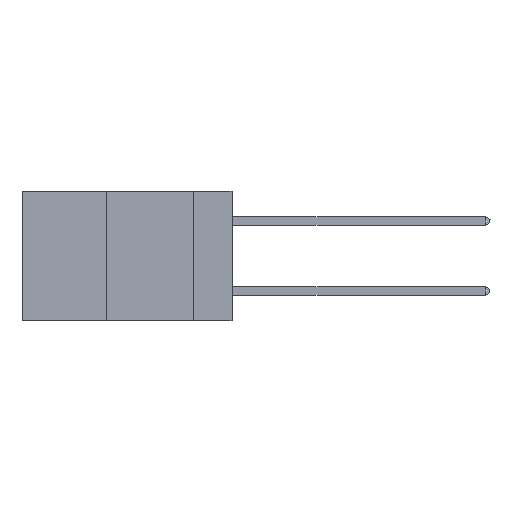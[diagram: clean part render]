
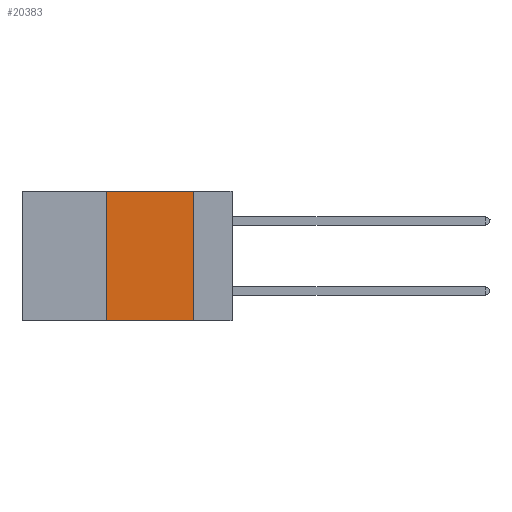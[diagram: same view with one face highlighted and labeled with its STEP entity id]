
A CAD part, left-side view. The second image highlights one B-rep face of the part: STEP entity #20383.
In plain terms, the highlighted planar face has unit normal (-1, 0, 0).
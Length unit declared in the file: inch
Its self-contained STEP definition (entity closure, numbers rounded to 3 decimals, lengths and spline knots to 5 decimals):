
#165 = EDGE_CURVE ( 'NONE', #16418, #5403, #18769, .T. ) ;
#1381 = CARTESIAN_POINT ( 'NONE',  ( 0., 0.6, 0. ) ) ;
#2147 = ORIENTED_EDGE ( 'NONE', *, *, #17951, .F. ) ;
#2774 = CARTESIAN_POINT ( 'NONE',  ( 0., 0.6, -0.37 ) ) ;
#3889 = VECTOR ( 'NONE', #14009, 39.37008 ) ;
#4138 = CARTESIAN_POINT ( 'NONE',  ( 0., 0.11, 0. ) ) ;
#4180 = ORIENTED_EDGE ( 'NONE', *, *, #7829, .F. ) ;
#4671 = VERTEX_POINT ( 'NONE', #11253 ) ;
#5403 = VERTEX_POINT ( 'NONE', #4138 ) ;
#6402 = CARTESIAN_POINT ( 'NONE',  ( 0., 0.11, -0.37 ) ) ;
#6785 = ORIENTED_EDGE ( 'NONE', *, *, #165, .F. ) ;
#6992 = VECTOR ( 'NONE', #8208, 39.37008 ) ;
#7829 = EDGE_CURVE ( 'NONE', #5403, #17338, #13339, .T. ) ;
#8042 = VECTOR ( 'NONE', #8101, 39.37008 ) ;
#8101 = DIRECTION ( 'NONE',  ( 0., 0., 1. ) ) ;
#8208 = DIRECTION ( 'NONE',  ( 0., -1., 0. ) ) ;
#8416 = DIRECTION ( 'NONE',  ( 0., 0., -1. ) ) ;
#8870 = EDGE_CURVE ( 'NONE', #4671, #17338, #15714, .T. ) ;
#9381 = ORIENTED_EDGE ( 'NONE', *, *, #8870, .T. ) ;
#9896 = FACE_OUTER_BOUND ( 'NONE', #21967, .T. ) ;
#10571 = CARTESIAN_POINT ( 'NONE',  ( 0., 0.11, 0. ) ) ;
#11253 = CARTESIAN_POINT ( 'NONE',  ( 0., 0.36, -0.37 ) ) ;
#12671 = CARTESIAN_POINT ( 'NONE',  ( 0., 0.36, 0. ) ) ;
#13225 = LINE ( 'NONE', #16712, #8042 ) ;
#13339 = LINE ( 'NONE', #10571, #3889 ) ;
#14009 = DIRECTION ( 'NONE',  ( 0., 0., -1. ) ) ;
#14230 = VECTOR ( 'NONE', #18761, 39.37008 ) ;
#15714 = LINE ( 'NONE', #2774, #6992 ) ;
#16225 = AXIS2_PLACEMENT_3D ( 'NONE', #17015, #18727, #8416 ) ;
#16418 = VERTEX_POINT ( 'NONE', #12671 ) ;
#16712 = CARTESIAN_POINT ( 'NONE',  ( 0., 0.36, 0. ) ) ;
#17015 = CARTESIAN_POINT ( 'NONE',  ( 0., 0.6, 0. ) ) ;
#17338 = VERTEX_POINT ( 'NONE', #6402 ) ;
#17951 = EDGE_CURVE ( 'NONE', #4671, #16418, #13225, .T. ) ;
#18727 = DIRECTION ( 'NONE',  ( 1., 0., 0. ) ) ;
#18761 = DIRECTION ( 'NONE',  ( 0., -1., 0. ) ) ;
#18769 = LINE ( 'NONE', #1381, #14230 ) ;
#20383 = ADVANCED_FACE ( 'NONE', ( #9896 ), #22050, .F. ) ;
#21967 = EDGE_LOOP ( 'NONE', ( #4180, #6785, #2147, #9381 ) ) ;
#22050 = PLANE ( 'NONE',  #16225 ) ;
